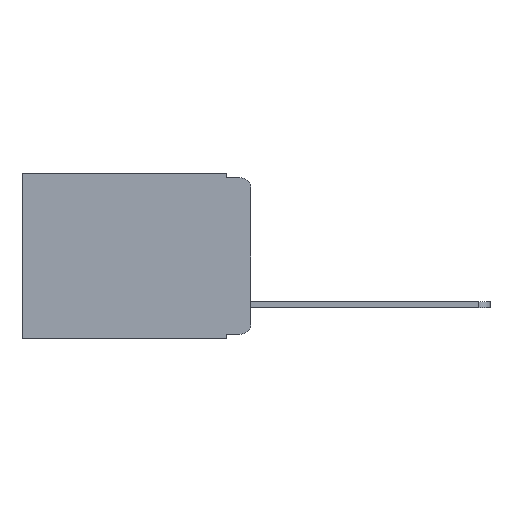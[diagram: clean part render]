
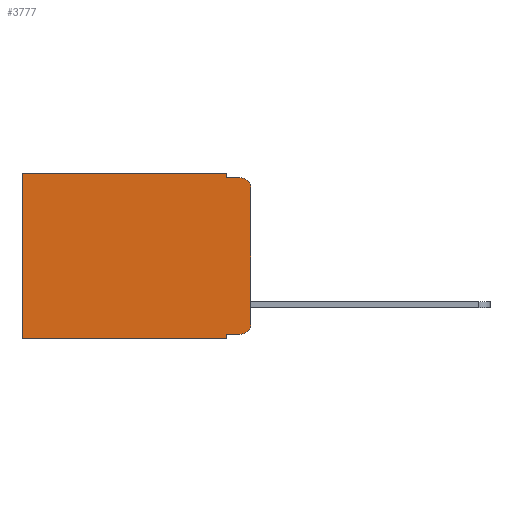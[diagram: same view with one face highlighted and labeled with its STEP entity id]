
A CAD part, left-side view. The second image highlights one B-rep face of the part: STEP entity #3777.
In plain terms, the highlighted planar face has unit normal (-1, 0, 0).
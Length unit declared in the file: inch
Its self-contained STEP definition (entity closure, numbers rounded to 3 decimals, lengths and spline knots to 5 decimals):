
#244 = CARTESIAN_POINT ( 'NONE',  ( 0.298, 0., -0.343 ) ) ;
#333 = VECTOR ( 'NONE', #3451, 39.37008 ) ;
#402 = ORIENTED_EDGE ( 'NONE', *, *, #6355, .F. ) ;
#596 = CARTESIAN_POINT ( 'NONE',  ( 0.298, 0., 0. ) ) ;
#609 = VERTEX_POINT ( 'NONE', #6237 ) ;
#706 = LINE ( 'NONE', #2676, #6789 ) ;
#724 = ORIENTED_EDGE ( 'NONE', *, *, #1114, .F. ) ;
#812 = CARTESIAN_POINT ( 'NONE',  ( 0.298, 0.051, -0.343 ) ) ;
#934 = ORIENTED_EDGE ( 'NONE', *, *, #9160, .T. ) ;
#987 = LINE ( 'NONE', #244, #6973 ) ;
#1114 = EDGE_CURVE ( 'NONE', #5880, #2664, #8524, .T. ) ;
#1154 = CARTESIAN_POINT ( 'NONE',  ( 0.298, 0.02, -0.313 ) ) ;
#1386 = FACE_OUTER_BOUND ( 'NONE', #2780, .T. ) ;
#1506 = CARTESIAN_POINT ( 'NONE',  ( 0.298, 0.473, 0. ) ) ;
#1898 = ORIENTED_EDGE ( 'NONE', *, *, #8016, .F. ) ;
#2036 = LINE ( 'NONE', #5672, #8648 ) ;
#2135 = DIRECTION ( 'NONE',  ( 1., 0., 0. ) ) ;
#2291 = VERTEX_POINT ( 'NONE', #2635 ) ;
#2423 = EDGE_CURVE ( 'NONE', #2291, #3140, #4818, .T. ) ;
#2464 = VERTEX_POINT ( 'NONE', #8262 ) ;
#2551 = LINE ( 'NONE', #3246, #10281 ) ;
#2634 = VERTEX_POINT ( 'NONE', #1506 ) ;
#2635 = CARTESIAN_POINT ( 'NONE',  ( 0.298, 0.02, -0.333 ) ) ;
#2664 = VERTEX_POINT ( 'NONE', #812 ) ;
#2676 = CARTESIAN_POINT ( 'NONE',  ( 0.298, 0.051, 0. ) ) ;
#2780 = EDGE_LOOP ( 'NONE', ( #402, #934, #9275, #1898, #6056, #10501, #6041, #724, #5980, #6535 ) ) ;
#3095 = EDGE_CURVE ( 'NONE', #2634, #2464, #2551, .T. ) ;
#3140 = VERTEX_POINT ( 'NONE', #6732 ) ;
#3185 = VERTEX_POINT ( 'NONE', #3538 ) ;
#3246 = CARTESIAN_POINT ( 'NONE',  ( 0.298, 0.473, 0. ) ) ;
#3267 = CIRCLE ( 'NONE', #6410, 0.02 ) ;
#3451 = DIRECTION ( 'NONE',  ( 0., 0., -1. ) ) ;
#3523 = CARTESIAN_POINT ( 'NONE',  ( 0.298, 0.051, -0.333 ) ) ;
#3538 = CARTESIAN_POINT ( 'NONE',  ( 0.298, 0.051, 0. ) ) ;
#3777 = ADVANCED_FACE ( 'NONE', ( #1386 ), #9353, .F. ) ;
#3785 = EDGE_CURVE ( 'NONE', #3185, #2634, #4156, .T. ) ;
#3796 = DIRECTION ( 'NONE',  ( 0., 1., 0. ) ) ;
#4103 = DIRECTION ( 'NONE',  ( 0., 0., -1. ) ) ;
#4156 = LINE ( 'NONE', #8435, #9411 ) ;
#4647 = VERTEX_POINT ( 'NONE', #5810 ) ;
#4818 = CIRCLE ( 'NONE', #10924, 0.02 ) ;
#4970 = CARTESIAN_POINT ( 'NONE',  ( 0.298, 0.02, -0.03 ) ) ;
#5092 = DIRECTION ( 'NONE',  ( 0., -1., 0. ) ) ;
#5672 = CARTESIAN_POINT ( 'NONE',  ( 0.298, 0.051, -0.333 ) ) ;
#5776 = DIRECTION ( 'NONE',  ( 0., 0., -1. ) ) ;
#5810 = CARTESIAN_POINT ( 'NONE',  ( 0.298, 0.051, -0.01 ) ) ;
#5817 = CARTESIAN_POINT ( 'NONE',  ( 0.298, 0.02, -0.01 ) ) ;
#5831 = DIRECTION ( 'NONE',  ( 0., 1., 0. ) ) ;
#5880 = VERTEX_POINT ( 'NONE', #3523 ) ;
#5944 = VECTOR ( 'NONE', #11256, 39.37008 ) ;
#5980 = ORIENTED_EDGE ( 'NONE', *, *, #9094, .T. ) ;
#6041 = ORIENTED_EDGE ( 'NONE', *, *, #7809, .F. ) ;
#6056 = ORIENTED_EDGE ( 'NONE', *, *, #3785, .T. ) ;
#6112 = DIRECTION ( 'NONE',  ( 0., 0., -1. ) ) ;
#6233 = VECTOR ( 'NONE', #10202, 39.37008 ) ;
#6237 = CARTESIAN_POINT ( 'NONE',  ( 0.298, 0., -0.03 ) ) ;
#6355 = EDGE_CURVE ( 'NONE', #609, #3140, #8747, .T. ) ;
#6410 = AXIS2_PLACEMENT_3D ( 'NONE', #4970, #8503, #4103 ) ;
#6535 = ORIENTED_EDGE ( 'NONE', *, *, #2423, .T. ) ;
#6732 = CARTESIAN_POINT ( 'NONE',  ( 0.298, 0., -0.313 ) ) ;
#6789 = VECTOR ( 'NONE', #11351, 39.37008 ) ;
#6973 = VECTOR ( 'NONE', #3796, 39.37008 ) ;
#7016 = VERTEX_POINT ( 'NONE', #5817 ) ;
#7154 = DIRECTION ( 'NONE',  ( -1., 0., 0. ) ) ;
#7568 = AXIS2_PLACEMENT_3D ( 'NONE', #596, #2135, #5776 ) ;
#7601 = CARTESIAN_POINT ( 'NONE',  ( 0.298, 0.051, -0.01 ) ) ;
#7809 = EDGE_CURVE ( 'NONE', #2664, #2464, #987, .T. ) ;
#8016 = EDGE_CURVE ( 'NONE', #3185, #4647, #706, .T. ) ;
#8262 = CARTESIAN_POINT ( 'NONE',  ( 0.298, 0.473, -0.343 ) ) ;
#8360 = LINE ( 'NONE', #7601, #6233 ) ;
#8435 = CARTESIAN_POINT ( 'NONE',  ( 0.298, 0., 0. ) ) ;
#8503 = DIRECTION ( 'NONE',  ( -1., 0., 0. ) ) ;
#8524 = LINE ( 'NONE', #9268, #5944 ) ;
#8648 = VECTOR ( 'NONE', #5092, 39.37008 ) ;
#8738 = EDGE_CURVE ( 'NONE', #4647, #7016, #8360, .T. ) ;
#8747 = LINE ( 'NONE', #11413, #333 ) ;
#9094 = EDGE_CURVE ( 'NONE', #5880, #2291, #2036, .T. ) ;
#9160 = EDGE_CURVE ( 'NONE', #609, #7016, #3267, .T. ) ;
#9268 = CARTESIAN_POINT ( 'NONE',  ( 0.298, 0.051, 0. ) ) ;
#9275 = ORIENTED_EDGE ( 'NONE', *, *, #8738, .F. ) ;
#9353 = PLANE ( 'NONE',  #7568 ) ;
#9411 = VECTOR ( 'NONE', #5831, 39.37008 ) ;
#9925 = DIRECTION ( 'NONE',  ( 0., 0., -1. ) ) ;
#10202 = DIRECTION ( 'NONE',  ( 0., -1., 0. ) ) ;
#10281 = VECTOR ( 'NONE', #6112, 39.37008 ) ;
#10501 = ORIENTED_EDGE ( 'NONE', *, *, #3095, .T. ) ;
#10924 = AXIS2_PLACEMENT_3D ( 'NONE', #1154, #7154, #9925 ) ;
#11256 = DIRECTION ( 'NONE',  ( 0., 0., -1. ) ) ;
#11351 = DIRECTION ( 'NONE',  ( 0., 0., -1. ) ) ;
#11413 = CARTESIAN_POINT ( 'NONE',  ( 0.298, 0., 0. ) ) ;
